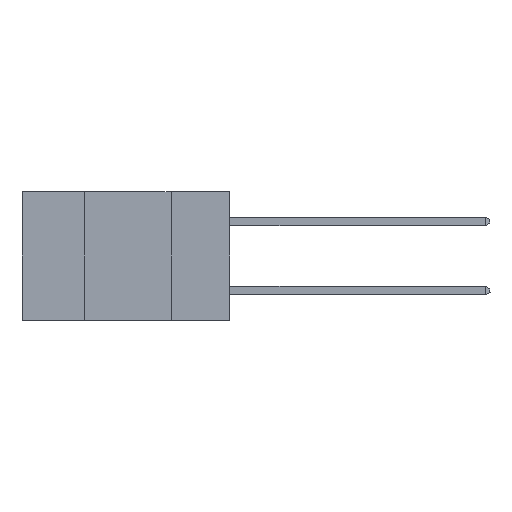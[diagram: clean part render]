
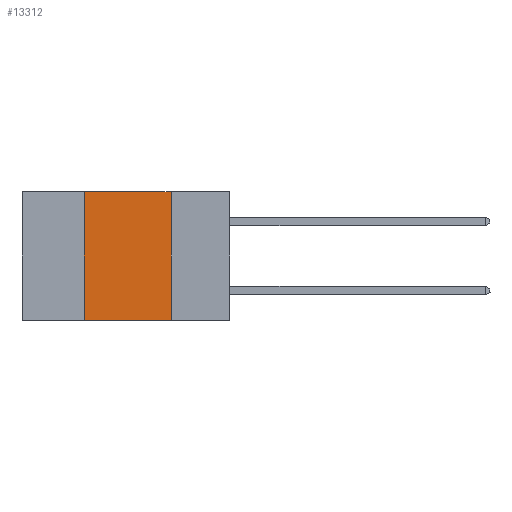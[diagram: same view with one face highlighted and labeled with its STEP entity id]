
A CAD part, left-side view. The second image highlights one B-rep face of the part: STEP entity #13312.
In plain terms, the highlighted planar face has unit normal (-1, 0, 0).
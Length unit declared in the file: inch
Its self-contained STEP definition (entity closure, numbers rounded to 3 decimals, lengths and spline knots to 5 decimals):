
#847 = EDGE_CURVE ( 'NONE', #13036, #6548, #5573, .T. ) ;
#2674 = LINE ( 'NONE', #10777, #7178 ) ;
#2912 = DIRECTION ( 'NONE',  ( 0., 0., -1. ) ) ;
#3495 = CARTESIAN_POINT ( 'NONE',  ( 0., 0.42, -0.37 ) ) ;
#3913 = CARTESIAN_POINT ( 'NONE',  ( 0., 0.6, 0. ) ) ;
#4253 = VERTEX_POINT ( 'NONE', #7134 ) ;
#4413 = EDGE_CURVE ( 'NONE', #13036, #11681, #2674, .T. ) ;
#4988 = CARTESIAN_POINT ( 'NONE',  ( 0., 0.17, -0.37 ) ) ;
#5573 = LINE ( 'NONE', #15949, #14012 ) ;
#6035 = EDGE_CURVE ( 'NONE', #4253, #11681, #19289, .T. ) ;
#6548 = VERTEX_POINT ( 'NONE', #10470 ) ;
#6990 = DIRECTION ( 'NONE',  ( 0., 0., 1. ) ) ;
#7134 = CARTESIAN_POINT ( 'NONE',  ( 0., 0.17, 0. ) ) ;
#7178 = VECTOR ( 'NONE', #16799, 39.37008 ) ;
#8770 = EDGE_LOOP ( 'NONE', ( #16594, #13306, #9455, #16205 ) ) ;
#8815 = LINE ( 'NONE', #3913, #15111 ) ;
#9455 = ORIENTED_EDGE ( 'NONE', *, *, #847, .F. ) ;
#10427 = CARTESIAN_POINT ( 'NONE',  ( 0., 0.17, 0. ) ) ;
#10470 = CARTESIAN_POINT ( 'NONE',  ( 0., 0.42, 0. ) ) ;
#10777 = CARTESIAN_POINT ( 'NONE',  ( 0., 0.6, -0.37 ) ) ;
#11084 = VECTOR ( 'NONE', #2912, 39.37008 ) ;
#11681 = VERTEX_POINT ( 'NONE', #4988 ) ;
#12128 = AXIS2_PLACEMENT_3D ( 'NONE', #12846, #12911, #14354 ) ;
#12846 = CARTESIAN_POINT ( 'NONE',  ( 0., 0.6, 0. ) ) ;
#12911 = DIRECTION ( 'NONE',  ( 1., 0., 0. ) ) ;
#13036 = VERTEX_POINT ( 'NONE', #3495 ) ;
#13306 = ORIENTED_EDGE ( 'NONE', *, *, #16660, .F. ) ;
#13312 = ADVANCED_FACE ( 'NONE', ( #13813 ), #18824, .F. ) ;
#13813 = FACE_OUTER_BOUND ( 'NONE', #8770, .T. ) ;
#14012 = VECTOR ( 'NONE', #6990, 39.37008 ) ;
#14328 = DIRECTION ( 'NONE',  ( 0., -1., 0. ) ) ;
#14354 = DIRECTION ( 'NONE',  ( 0., 0., -1. ) ) ;
#15111 = VECTOR ( 'NONE', #14328, 39.37008 ) ;
#15949 = CARTESIAN_POINT ( 'NONE',  ( 0., 0.42, 0. ) ) ;
#16205 = ORIENTED_EDGE ( 'NONE', *, *, #4413, .T. ) ;
#16594 = ORIENTED_EDGE ( 'NONE', *, *, #6035, .F. ) ;
#16660 = EDGE_CURVE ( 'NONE', #6548, #4253, #8815, .T. ) ;
#16799 = DIRECTION ( 'NONE',  ( 0., -1., 0. ) ) ;
#18824 = PLANE ( 'NONE',  #12128 ) ;
#19289 = LINE ( 'NONE', #10427, #11084 ) ;
